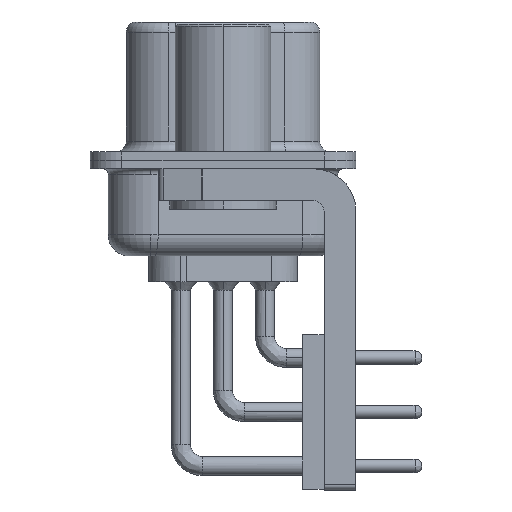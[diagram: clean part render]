
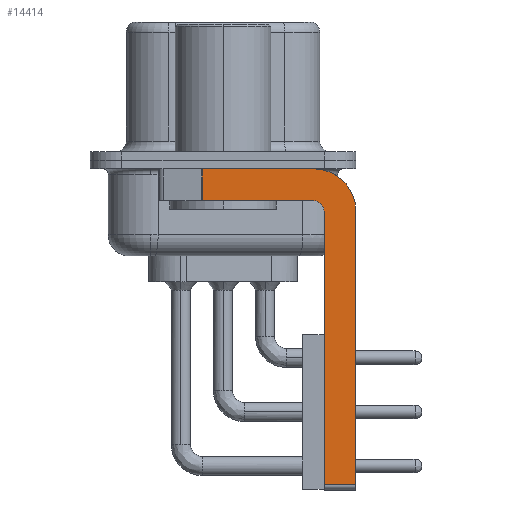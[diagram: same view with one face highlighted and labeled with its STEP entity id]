
A CAD part, left-side view. The second image highlights one B-rep face of the part: STEP entity #14414.
In plain terms, the highlighted planar face has unit normal (-1, 0, 0).
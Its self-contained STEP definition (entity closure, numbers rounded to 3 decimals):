
#701 = AXIS2_PLACEMENT_3D ( 'NONE', #8154, #25795, #10686 ) ;
#955 = EDGE_CURVE ( 'NONE', #18931, #16376, #11959, .T. ) ;
#1012 = DIRECTION ( 'NONE',  ( 0., -1., 0. ) ) ;
#1169 = ORIENTED_EDGE ( 'NONE', *, *, #11148, .F. ) ;
#1867 = CIRCLE ( 'NONE', #13276, 2. ) ;
#1909 = CARTESIAN_POINT ( 'NONE',  ( -2.9, 0.978, -0.4 ) ) ;
#2080 = EDGE_CURVE ( 'NONE', #25403, #16376, #32361, .T. ) ;
#2603 = LINE ( 'NONE', #26341, #15255 ) ;
#3519 = CARTESIAN_POINT ( 'NONE',  ( -2.9, 0.978, -1.9 ) ) ;
#3531 = LINE ( 'NONE', #25956, #22901 ) ;
#3939 = VERTEX_POINT ( 'NONE', #5705 ) ;
#4445 = ORIENTED_EDGE ( 'NONE', *, *, #22867, .F. ) ;
#5349 = CARTESIAN_POINT ( 'NONE',  ( -2.9, -4.25, -15.25 ) ) ;
#5705 = CARTESIAN_POINT ( 'NONE',  ( -2.9, -4.25, -1.9 ) ) ;
#5794 = DIRECTION ( 'NONE',  ( 0., -1., 0. ) ) ;
#5970 = CIRCLE ( 'NONE', #701, 0.5 ) ;
#6058 = CARTESIAN_POINT ( 'NONE',  ( -2.9, -4.25, -2.4 ) ) ;
#7068 = ORIENTED_EDGE ( 'NONE', *, *, #955, .T. ) ;
#8154 = CARTESIAN_POINT ( 'NONE',  ( -2.9, -4.25, -2.4 ) ) ;
#8245 = EDGE_CURVE ( 'NONE', #18931, #26179, #3531, .T. ) ;
#8257 = CARTESIAN_POINT ( 'NONE',  ( -2.9, -4.25, -0.4 ) ) ;
#9275 = ORIENTED_EDGE ( 'NONE', *, *, #8245, .F. ) ;
#9652 = CARTESIAN_POINT ( 'NONE',  ( -2.9, 0.978, -1.9 ) ) ;
#10114 = EDGE_CURVE ( 'NONE', #21118, #25403, #1867, .T. ) ;
#10686 = DIRECTION ( 'NONE',  ( 0., 0., 1. ) ) ;
#11148 = EDGE_CURVE ( 'NONE', #18050, #21118, #2603, .T. ) ;
#11157 = DIRECTION ( 'NONE',  ( 1., 0., 0. ) ) ;
#11405 = VECTOR ( 'NONE', #24589, 1000. ) ;
#11895 = CARTESIAN_POINT ( 'NONE',  ( -2.9, -4.25, -2.4 ) ) ;
#11924 = VERTEX_POINT ( 'NONE', #9652 ) ;
#11959 = LINE ( 'NONE', #5349, #17114 ) ;
#13276 = AXIS2_PLACEMENT_3D ( 'NONE', #11895, #29503, #14426 ) ;
#13280 = DIRECTION ( 'NONE',  ( 0., 0., 1. ) ) ;
#14281 = VECTOR ( 'NONE', #28639, 1000. ) ;
#14414 = ADVANCED_FACE ( 'NONE', ( #17748 ), #26257, .F. ) ;
#14426 = DIRECTION ( 'NONE',  ( 0., 0., -1. ) ) ;
#14643 = EDGE_CURVE ( 'NONE', #3939, #11924, #31478, .T. ) ;
#15062 = LINE ( 'NONE', #3519, #14281 ) ;
#15255 = VECTOR ( 'NONE', #1012, 1000. ) ;
#16073 = ORIENTED_EDGE ( 'NONE', *, *, #2080, .F. ) ;
#16376 = VERTEX_POINT ( 'NONE', #25627 ) ;
#17114 = VECTOR ( 'NONE', #5794, 1000. ) ;
#17697 = ORIENTED_EDGE ( 'NONE', *, *, #22354, .T. ) ;
#17748 = FACE_OUTER_BOUND ( 'NONE', #21602, .T. ) ;
#18050 = VERTEX_POINT ( 'NONE', #1909 ) ;
#18931 = VERTEX_POINT ( 'NONE', #28555 ) ;
#19674 = ORIENTED_EDGE ( 'NONE', *, *, #14643, .F. ) ;
#21118 = VERTEX_POINT ( 'NONE', #8257 ) ;
#21318 = ORIENTED_EDGE ( 'NONE', *, *, #10114, .F. ) ;
#21602 = EDGE_LOOP ( 'NONE', ( #1169, #17697, #19674, #4445, #9275, #7068, #16073, #21318 ) ) ;
#22354 = EDGE_CURVE ( 'NONE', #18050, #11924, #15062, .T. ) ;
#22730 = CARTESIAN_POINT ( 'NONE',  ( -2.9, -6.25, -2.4 ) ) ;
#22867 = EDGE_CURVE ( 'NONE', #26179, #3939, #5970, .T. ) ;
#22901 = VECTOR ( 'NONE', #13280, 1000. ) ;
#24589 = DIRECTION ( 'NONE',  ( 0., 1., 0. ) ) ;
#24890 = VECTOR ( 'NONE', #26133, 1000. ) ;
#25403 = VERTEX_POINT ( 'NONE', #22730 ) ;
#25627 = CARTESIAN_POINT ( 'NONE',  ( -2.9, -6.25, -15.25 ) ) ;
#25795 = DIRECTION ( 'NONE',  ( -1., 0., 0. ) ) ;
#25956 = CARTESIAN_POINT ( 'NONE',  ( -2.9, -4.75, -15.5 ) ) ;
#26133 = DIRECTION ( 'NONE',  ( 0., 0., -1. ) ) ;
#26179 = VERTEX_POINT ( 'NONE', #28070 ) ;
#26257 = PLANE ( 'NONE',  #30689 ) ;
#26341 = CARTESIAN_POINT ( 'NONE',  ( -2.9, 3., -0.4 ) ) ;
#28070 = CARTESIAN_POINT ( 'NONE',  ( -2.9, -4.75, -2.4 ) ) ;
#28345 = CARTESIAN_POINT ( 'NONE',  ( -2.9, -6.25, -2.4 ) ) ;
#28555 = CARTESIAN_POINT ( 'NONE',  ( -2.9, -4.75, -15.25 ) ) ;
#28639 = DIRECTION ( 'NONE',  ( 0., 0., -1. ) ) ;
#28749 = DIRECTION ( 'NONE',  ( 0., 0., -1. ) ) ;
#29503 = DIRECTION ( 'NONE',  ( 1., 0., 0. ) ) ;
#30689 = AXIS2_PLACEMENT_3D ( 'NONE', #6058, #11157, #28749 ) ;
#31478 = LINE ( 'NONE', #32598, #11405 ) ;
#32361 = LINE ( 'NONE', #28345, #24890 ) ;
#32598 = CARTESIAN_POINT ( 'NONE',  ( -2.9, -4.25, -1.9 ) ) ;
